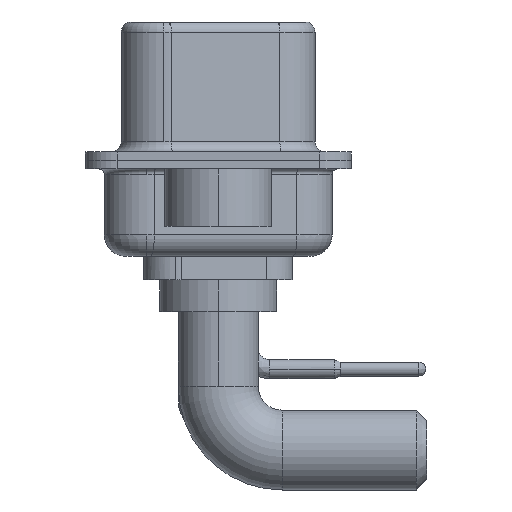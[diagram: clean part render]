
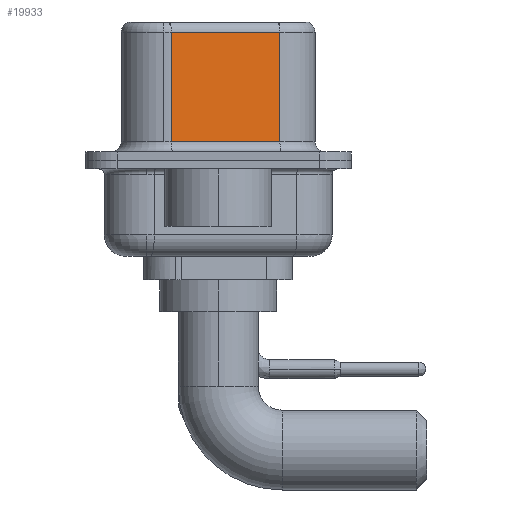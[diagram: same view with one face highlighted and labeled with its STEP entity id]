
A CAD part, left-side view. The second image highlights one B-rep face of the part: STEP entity #19933.
In plain terms, the highlighted planar face has unit normal (-0.985, -0.174, 0).
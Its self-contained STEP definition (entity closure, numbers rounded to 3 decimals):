
#6 = CARTESIAN_POINT ( 'NONE',  ( 3.68, 2.203, 6.02 ) ) ;
#985 = LINE ( 'NONE', #19929, #6539 ) ;
#1377 = CARTESIAN_POINT ( 'NONE',  ( 4.58, -2.897, 6.52 ) ) ;
#1714 = VERTEX_POINT ( 'NONE', #3237 ) ;
#3237 = CARTESIAN_POINT ( 'NONE',  ( 4.58, -2.897, 0.9 ) ) ;
#4324 = CARTESIAN_POINT ( 'NONE',  ( 3.68, 2.203, 0.9 ) ) ;
#4530 = EDGE_CURVE ( 'NONE', #23528, #24970, #16003, .T. ) ;
#4802 = AXIS2_PLACEMENT_3D ( 'NONE', #1377, #22721, #23147 ) ;
#5430 = DIRECTION ( 'NONE',  ( 0.174, -0.985, 0. ) ) ;
#5463 = PLANE ( 'NONE',  #4802 ) ;
#6539 = VECTOR ( 'NONE', #16096, 1000. ) ;
#6790 = ORIENTED_EDGE ( 'NONE', *, *, #25879, .F. ) ;
#10930 = VECTOR ( 'NONE', #14209, 1000. ) ;
#11381 = EDGE_LOOP ( 'NONE', ( #6790, #25768, #14560, #25482 ) ) ;
#11513 = CARTESIAN_POINT ( 'NONE',  ( 3.68, 2.203, 6.52 ) ) ;
#11676 = EDGE_CURVE ( 'NONE', #16754, #23528, #985, .T. ) ;
#12099 = LINE ( 'NONE', #16031, #10930 ) ;
#13149 = VECTOR ( 'NONE', #18543, 1000. ) ;
#14209 = DIRECTION ( 'NONE',  ( 0., 0., -1. ) ) ;
#14560 = ORIENTED_EDGE ( 'NONE', *, *, #4530, .T. ) ;
#16003 = LINE ( 'NONE', #11513, #13149 ) ;
#16031 = CARTESIAN_POINT ( 'NONE',  ( 4.58, -2.897, 6.52 ) ) ;
#16096 = DIRECTION ( 'NONE',  ( -0.174, 0.985, 0. ) ) ;
#16754 = VERTEX_POINT ( 'NONE', #16764 ) ;
#16764 = CARTESIAN_POINT ( 'NONE',  ( 4.58, -2.897, 6.02 ) ) ;
#18543 = DIRECTION ( 'NONE',  ( 0., 0., -1. ) ) ;
#19707 = VECTOR ( 'NONE', #5430, 1000. ) ;
#19929 = CARTESIAN_POINT ( 'NONE',  ( 4.58, -2.897, 6.02 ) ) ;
#19933 = ADVANCED_FACE ( 'NONE', ( #24857 ), #5463, .F. ) ;
#20405 = LINE ( 'NONE', #27383, #19707 ) ;
#20468 = EDGE_CURVE ( 'NONE', #24970, #1714, #20405, .T. ) ;
#22721 = DIRECTION ( 'NONE',  ( 0.985, 0.174, 0. ) ) ;
#23147 = DIRECTION ( 'NONE',  ( -0.174, 0.985, 0. ) ) ;
#23528 = VERTEX_POINT ( 'NONE', #6 ) ;
#24857 = FACE_OUTER_BOUND ( 'NONE', #11381, .T. ) ;
#24970 = VERTEX_POINT ( 'NONE', #4324 ) ;
#25482 = ORIENTED_EDGE ( 'NONE', *, *, #20468, .T. ) ;
#25768 = ORIENTED_EDGE ( 'NONE', *, *, #11676, .T. ) ;
#25879 = EDGE_CURVE ( 'NONE', #16754, #1714, #12099, .T. ) ;
#27383 = CARTESIAN_POINT ( 'NONE',  ( 4.58, -2.897, 0.9 ) ) ;
